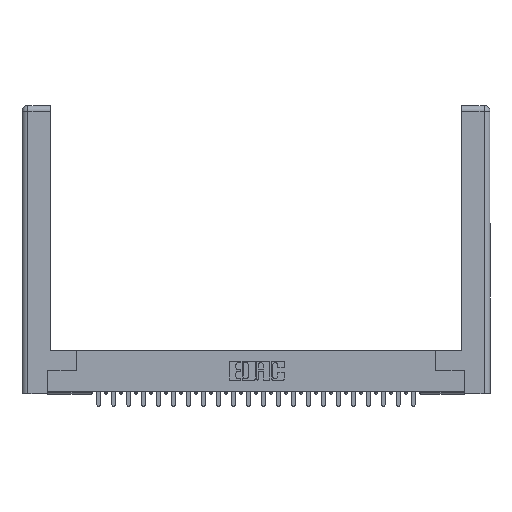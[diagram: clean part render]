
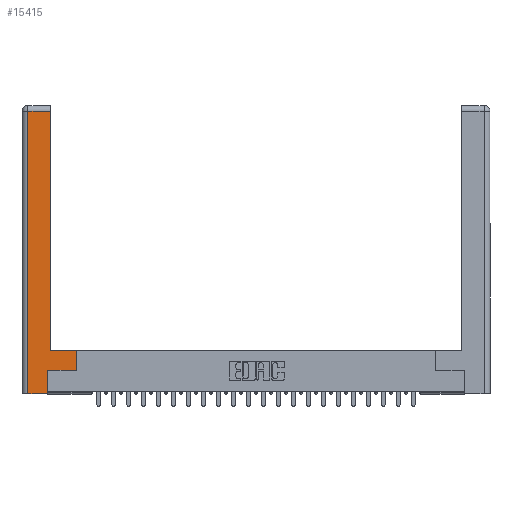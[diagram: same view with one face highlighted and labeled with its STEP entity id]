
A CAD part, top view. The second image highlights one B-rep face of the part: STEP entity #15415.
In plain terms, the highlighted planar face has unit normal (0, 0, 1).
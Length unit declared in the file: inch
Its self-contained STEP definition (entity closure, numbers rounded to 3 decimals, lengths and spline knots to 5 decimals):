
#156 = VERTEX_POINT ( 'NONE', #13468 ) ;
#1271 = DIRECTION ( 'NONE',  ( 0., 1., 0. ) ) ;
#1730 = VERTEX_POINT ( 'NONE', #6532 ) ;
#2781 = VECTOR ( 'NONE', #5401, 39.37008 ) ;
#3212 = CARTESIAN_POINT ( 'NONE',  ( 0.265, 0., 0. ) ) ;
#3249 = DIRECTION ( 'NONE',  ( 1., 0., 0. ) ) ;
#3481 = VECTOR ( 'NONE', #11777, 39.37008 ) ;
#3556 = EDGE_CURVE ( 'NONE', #18141, #7219, #8077, .T. ) ;
#3925 = CARTESIAN_POINT ( 'NONE',  ( 0.265, 0., 0. ) ) ;
#4095 = DIRECTION ( 'NONE',  ( 1., 0., 0. ) ) ;
#4097 = VECTOR ( 'NONE', #22680, 39.37008 ) ;
#4378 = VERTEX_POINT ( 'NONE', #7723 ) ;
#4942 = CARTESIAN_POINT ( 'NONE',  ( 0.265, 0.245, 0. ) ) ;
#5401 = DIRECTION ( 'NONE',  ( 0., 1., 0. ) ) ;
#6532 = CARTESIAN_POINT ( 'NONE',  ( 0.0615, 2.94, 0. ) ) ;
#6814 = ORIENTED_EDGE ( 'NONE', *, *, #12533, .T. ) ;
#6840 = LINE ( 'NONE', #9141, #20161 ) ;
#7219 = VERTEX_POINT ( 'NONE', #10286 ) ;
#7723 = CARTESIAN_POINT ( 'NONE',  ( 0.565, 0.45, 0. ) ) ;
#7751 = VECTOR ( 'NONE', #4095, 39.37008 ) ;
#7771 = FACE_OUTER_BOUND ( 'NONE', #18825, .T. ) ;
#8077 = LINE ( 'NONE', #25150, #2781 ) ;
#9141 = CARTESIAN_POINT ( 'NONE',  ( 0.565, 0.45, 0. ) ) ;
#9384 = LINE ( 'NONE', #13757, #3481 ) ;
#9456 = ORIENTED_EDGE ( 'NONE', *, *, #11183, .T. ) ;
#9528 = DIRECTION ( 'NONE',  ( -1., 0., 0. ) ) ;
#9692 = PLANE ( 'NONE',  #19841 ) ;
#10286 = CARTESIAN_POINT ( 'NONE',  ( 0.295, 2.94, 0. ) ) ;
#10323 = VECTOR ( 'NONE', #3249, 39.37008 ) ;
#10650 = ORIENTED_EDGE ( 'NONE', *, *, #11293, .T. ) ;
#11183 = EDGE_CURVE ( 'NONE', #23076, #17574, #14916, .T. ) ;
#11293 = EDGE_CURVE ( 'NONE', #17574, #156, #19288, .T. ) ;
#11777 = DIRECTION ( 'NONE',  ( 0., -1., 0. ) ) ;
#11795 = DIRECTION ( 'NONE',  ( 0., 0., -1. ) ) ;
#12533 = EDGE_CURVE ( 'NONE', #17915, #23076, #19843, .T. ) ;
#13146 = CARTESIAN_POINT ( 'NONE',  ( 0.565, 0.245, 0. ) ) ;
#13468 = CARTESIAN_POINT ( 'NONE',  ( 0.565, 0.245, 0. ) ) ;
#13757 = CARTESIAN_POINT ( 'NONE',  ( 0.0615, 0., 0. ) ) ;
#14026 = ORIENTED_EDGE ( 'NONE', *, *, #24007, .T. ) ;
#14747 = CARTESIAN_POINT ( 'NONE',  ( 0.265, 0.245, 0. ) ) ;
#14916 = LINE ( 'NONE', #4942, #4097 ) ;
#15415 = ADVANCED_FACE ( 'NONE', ( #7771 ), #9692, .F. ) ;
#16999 = CARTESIAN_POINT ( 'NONE',  ( 0.295, 0.45, 0. ) ) ;
#17000 = LINE ( 'NONE', #25328, #19492 ) ;
#17173 = DIRECTION ( 'NONE',  ( -1., 0., 0. ) ) ;
#17574 = VERTEX_POINT ( 'NONE', #14747 ) ;
#17915 = VERTEX_POINT ( 'NONE', #23495 ) ;
#18141 = VERTEX_POINT ( 'NONE', #16999 ) ;
#18825 = EDGE_LOOP ( 'NONE', ( #18873, #14026, #20300, #6814, #9456, #10650, #19614, #25545 ) ) ;
#18873 = ORIENTED_EDGE ( 'NONE', *, *, #3556, .T. ) ;
#19249 = CARTESIAN_POINT ( 'NONE',  ( 0.0615, 2.94, 0. ) ) ;
#19288 = LINE ( 'NONE', #13146, #10323 ) ;
#19492 = VECTOR ( 'NONE', #9528, 39.37008 ) ;
#19614 = ORIENTED_EDGE ( 'NONE', *, *, #23404, .T. ) ;
#19822 = EDGE_CURVE ( 'NONE', #1730, #17915, #9384, .T. ) ;
#19841 = AXIS2_PLACEMENT_3D ( 'NONE', #25575, #11795, #25675 ) ;
#19843 = LINE ( 'NONE', #3925, #7751 ) ;
#20161 = VECTOR ( 'NONE', #1271, 39.37008 ) ;
#20300 = ORIENTED_EDGE ( 'NONE', *, *, #19822, .T. ) ;
#22320 = VECTOR ( 'NONE', #17173, 39.37008 ) ;
#22680 = DIRECTION ( 'NONE',  ( 0., 1., 0. ) ) ;
#23076 = VERTEX_POINT ( 'NONE', #3212 ) ;
#23404 = EDGE_CURVE ( 'NONE', #156, #4378, #6840, .T. ) ;
#23495 = CARTESIAN_POINT ( 'NONE',  ( 0.0615, 0., 0. ) ) ;
#24007 = EDGE_CURVE ( 'NONE', #7219, #1730, #25437, .T. ) ;
#24161 = EDGE_CURVE ( 'NONE', #4378, #18141, #17000, .T. ) ;
#25150 = CARTESIAN_POINT ( 'NONE',  ( 0.295, 3., 0. ) ) ;
#25328 = CARTESIAN_POINT ( 'NONE',  ( 0.295, 0.45, 0. ) ) ;
#25437 = LINE ( 'NONE', #19249, #22320 ) ;
#25545 = ORIENTED_EDGE ( 'NONE', *, *, #24161, .T. ) ;
#25575 = CARTESIAN_POINT ( 'NONE',  ( 0., 0., 0. ) ) ;
#25675 = DIRECTION ( 'NONE',  ( -1., 0., 0. ) ) ;
